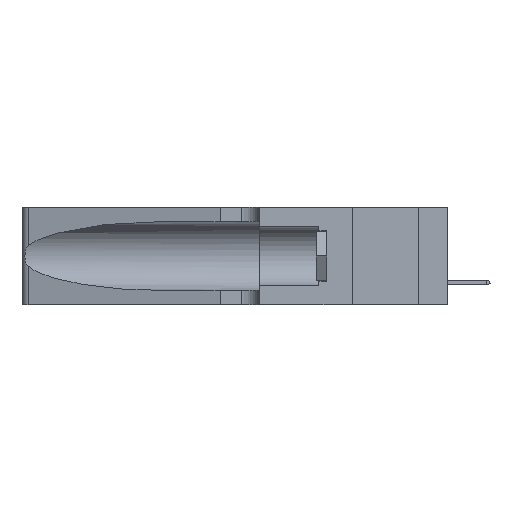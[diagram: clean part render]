
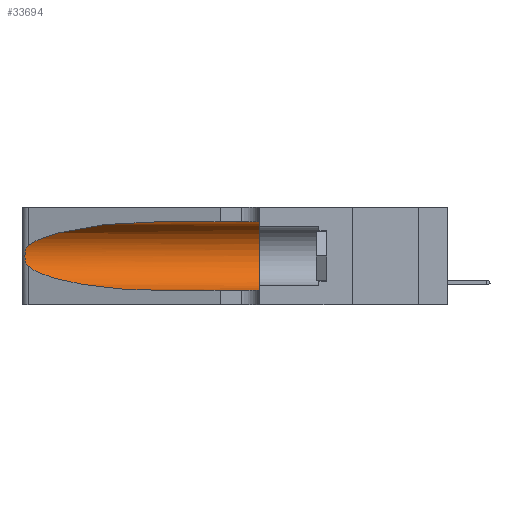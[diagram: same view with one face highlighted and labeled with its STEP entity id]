
A CAD part, left-side view. The second image highlights one B-rep face of the part: STEP entity #33694.
In plain terms, the highlighted cylindrical face has radius 3.308 mm (diameter 6.617 mm), a partial arc.
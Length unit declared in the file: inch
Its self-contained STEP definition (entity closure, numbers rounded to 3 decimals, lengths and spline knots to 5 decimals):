
#824 = CARTESIAN_POINT ( 'NONE',  ( 0.25789, 1.23486, 0.15765 ) ) ;
#882 = ORIENTED_EDGE ( 'NONE', *, *, #20993, .T. ) ;
#1510 = CARTESIAN_POINT ( 'NONE',  ( 0.25487, 1.22718, 0.22369 ) ) ;
#2422 =( BOUNDED_CURVE ( )  B_SPLINE_CURVE ( 3, ( #11492, #39298, #42746, #1510 ),
 .UNSPECIFIED., .F., .F. ) 
 B_SPLINE_CURVE_WITH_KNOTS ( ( 4, 4 ),
 ( 1.5708, 2.84003 ),
 .UNSPECIFIED. ) 
 CURVE ( )  GEOMETRIC_REPRESENTATION_ITEM ( )  RATIONAL_B_SPLINE_CURVE ( ( 1., 0.87, 0.87, 1. ) ) 
 REPRESENTATION_ITEM ( '' )  );
#2773 = CARTESIAN_POINT ( 'NONE',  ( 0.25555, 1.22994, 0.2215 ) ) ;
#3019 = VERTEX_POINT ( 'NONE', #35869 ) ;
#4176 = CARTESIAN_POINT ( 'NONE',  ( 0.25487, 1.22718, 0.14631 ) ) ;
#4308 = ORIENTED_EDGE ( 'NONE', *, *, #28550, .T. ) ;
#6241 = CARTESIAN_POINT ( 'NONE',  ( 0.25639, 1.23184, 0.21858 ) ) ;
#6452 = ORIENTED_EDGE ( 'NONE', *, *, #38716, .T. ) ;
#6454 = VECTOR ( 'NONE', #44098, 39.37008 ) ;
#6967 = LINE ( 'NONE', #16652, #6454 ) ;
#7421 = VERTEX_POINT ( 'NONE', #7876 ) ;
#7876 = CARTESIAN_POINT ( 'NONE',  ( 0.1305, 0.72297, 0.31525 ) ) ;
#10390 = CARTESIAN_POINT ( 'NONE',  ( 0.1305, 0.35, 0.31525 ) ) ;
#10759 = VERTEX_POINT ( 'NONE', #19164 ) ;
#11372 = CARTESIAN_POINT ( 'NONE',  ( 0.25487, 1.22718, 0.14631 ) ) ;
#11439 = CARTESIAN_POINT ( 'NONE',  ( 0.25555, 1.22993, 0.14849 ) ) ;
#11492 = CARTESIAN_POINT ( 'NONE',  ( 0.1305, 0.72297, 0.31525 ) ) ;
#11595 = EDGE_LOOP ( 'NONE', ( #4308, #6452, #33722, #882, #35898, #32801 ) ) ;
#11660 = LINE ( 'NONE', #21246, #43432 ) ;
#12998 = AXIS2_PLACEMENT_3D ( 'NONE', #28479, #34856, #31657 ) ;
#14158 = DIRECTION ( 'NONE',  ( 0., -1., 0. ) ) ;
#16086 = DIRECTION ( 'NONE',  ( 0., 1., 0. ) ) ;
#16652 = CARTESIAN_POINT ( 'NONE',  ( 0.1305, 1.61858, 0.05475 ) ) ;
#16850 = VERTEX_POINT ( 'NONE', #17196 ) ;
#17046 = CARTESIAN_POINT ( 'NONE',  ( 0.26075, 1.23896, 0.178 ) ) ;
#17196 = CARTESIAN_POINT ( 'NONE',  ( 0.25487, 1.22718, 0.14631 ) ) ;
#17724 = CARTESIAN_POINT ( 'NONE',  ( 0.25639, 1.23186, 0.15144 ) ) ;
#17770 = CIRCLE ( 'NONE', #33377, 0.13025 ) ;
#17802 = CARTESIAN_POINT ( 'NONE',  ( 0.1305, 0.72297, 0.05475 ) ) ;
#18378 = CARTESIAN_POINT ( 'NONE',  ( 0.1305, 0.35, 0.05475 ) ) ;
#18788 = DIRECTION ( 'NONE',  ( 0., 0., 1. ) ) ;
#18955 =( BOUNDED_CURVE ( )  B_SPLINE_CURVE ( 3, ( #11372, #21855, #28476, #17802 ),
 .UNSPECIFIED., .F., .F. ) 
 B_SPLINE_CURVE_WITH_KNOTS ( ( 4, 4 ),
 ( 3.44316, 4.71239 ),
 .UNSPECIFIED. ) 
 CURVE ( )  GEOMETRIC_REPRESENTATION_ITEM ( )  RATIONAL_B_SPLINE_CURVE ( ( 1., 0.87, 0.87, 1. ) ) 
 REPRESENTATION_ITEM ( '' )  );
#19164 = CARTESIAN_POINT ( 'NONE',  ( 0.25487, 1.22718, 0.22369 ) ) ;
#19929 = EDGE_CURVE ( 'NONE', #41662, #23244, #17770, .T. ) ;
#20993 = EDGE_CURVE ( 'NONE', #3019, #23244, #6967, .T. ) ;
#21246 = CARTESIAN_POINT ( 'NONE',  ( 0.1305, 1.61858, 0.31525 ) ) ;
#21373 = CYLINDRICAL_SURFACE ( 'NONE', #12998, 0.13025 ) ;
#21855 = CARTESIAN_POINT ( 'NONE',  ( 0.2373, 1.15595, 0.08982 ) ) ;
#23244 = VERTEX_POINT ( 'NONE', #18378 ) ;
#23842 = CARTESIAN_POINT ( 'NONE',  ( 0.25854, 1.2359, 0.20912 ) ) ;
#24399 = CARTESIAN_POINT ( 'NONE',  ( 0.25787, 1.23484, 0.2124 ) ) ;
#28476 = CARTESIAN_POINT ( 'NONE',  ( 0.18966, 0.96281, 0.05475 ) ) ;
#28479 = CARTESIAN_POINT ( 'NONE',  ( 0.1305, 1.61858, 0.185 ) ) ;
#28550 = EDGE_CURVE ( 'NONE', #7421, #10759, #2422, .T. ) ;
#30637 = FACE_OUTER_BOUND ( 'NONE', #11595, .T. ) ;
#30774 = CARTESIAN_POINT ( 'NONE',  ( 0.26018, 1.23835, 0.19895 ) ) ;
#31657 = DIRECTION ( 'NONE',  ( 0., 0., -1. ) ) ;
#32801 = ORIENTED_EDGE ( 'NONE', *, *, #43642, .F. ) ;
#33377 = AXIS2_PLACEMENT_3D ( 'NONE', #40040, #16086, #18788 ) ;
#33694 = ADVANCED_FACE ( 'NONE', ( #30637 ), #21373, .F. ) ;
#33722 = ORIENTED_EDGE ( 'NONE', *, *, #34287, .T. ) ;
#34287 = EDGE_CURVE ( 'NONE', #16850, #3019, #18955, .T. ) ;
#34856 = DIRECTION ( 'NONE',  ( 0., -1., 0. ) ) ;
#34927 = CARTESIAN_POINT ( 'NONE',  ( 0.25856, 1.23593, 0.16098 ) ) ;
#35869 = CARTESIAN_POINT ( 'NONE',  ( 0.1305, 0.72297, 0.05475 ) ) ;
#35898 = ORIENTED_EDGE ( 'NONE', *, *, #19929, .F. ) ;
#36939 = CARTESIAN_POINT ( 'NONE',  ( 0.25487, 1.22718, 0.22369 ) ) ;
#37698 = CARTESIAN_POINT ( 'NONE',  ( 0.26075, 1.23896, 0.19203 ) ) ;
#38716 = EDGE_CURVE ( 'NONE', #10759, #16850, #42944, .T. ) ;
#39298 = CARTESIAN_POINT ( 'NONE',  ( 0.18966, 0.96281, 0.31525 ) ) ;
#40040 = CARTESIAN_POINT ( 'NONE',  ( 0.1305, 0.35, 0.185 ) ) ;
#41138 = CARTESIAN_POINT ( 'NONE',  ( 0.26017, 1.23833, 0.17102 ) ) ;
#41662 = VERTEX_POINT ( 'NONE', #10390 ) ;
#42746 = CARTESIAN_POINT ( 'NONE',  ( 0.2373, 1.15595, 0.28018 ) ) ;
#42944 = B_SPLINE_CURVE_WITH_KNOTS ( 'NONE', 3,
 ( #36939, #2773, #6241, #24399, #23842, #30774, #37698, #17046, #41138, #34927, #824, #17724, #11439, #4176 ),
 .UNSPECIFIED., .F., .F.,
 ( 4, 2, 2, 2, 2, 2, 4 ),
 ( 0., 0.00027, 0.00053, 0.00107, 0.0016, 0.00187, 0.00214 ),
 .UNSPECIFIED. ) ;
#43432 = VECTOR ( 'NONE', #14158, 39.37008 ) ;
#43642 = EDGE_CURVE ( 'NONE', #7421, #41662, #11660, .T. ) ;
#44098 = DIRECTION ( 'NONE',  ( 0., -1., 0. ) ) ;
